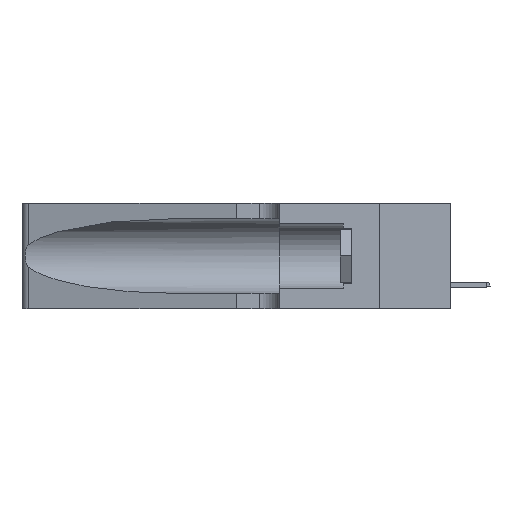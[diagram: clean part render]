
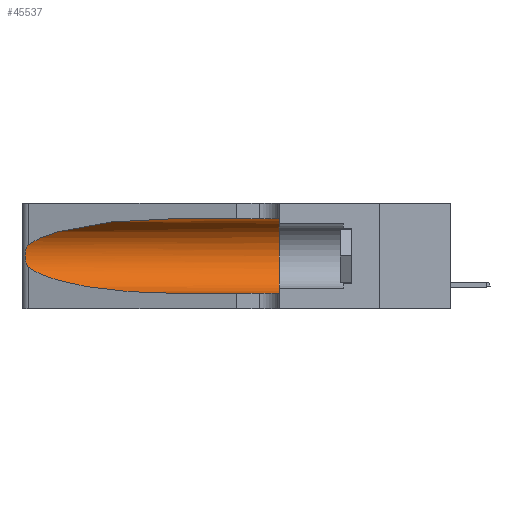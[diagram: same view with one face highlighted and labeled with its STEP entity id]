
A CAD part, left-side view. The second image highlights one B-rep face of the part: STEP entity #45537.
In plain terms, the highlighted cylindrical face has radius 3.308 mm (diameter 6.617 mm), a partial arc.
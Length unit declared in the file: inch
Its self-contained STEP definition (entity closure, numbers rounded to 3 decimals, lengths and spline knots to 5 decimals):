
#4463 = DIRECTION ( 'NONE',  ( 0., 0., -1. ) ) ;
#5229 =( BOUNDED_CURVE ( )  B_SPLINE_CURVE ( 3, ( #36028, #36274, #9947, #17600 ),
 .UNSPECIFIED., .F., .T. ) 
 B_SPLINE_CURVE_WITH_KNOTS ( ( 4, 4 ),
 ( 1.5708, 2.84003 ),
 .UNSPECIFIED. ) 
 CURVE ( )  GEOMETRIC_REPRESENTATION_ITEM ( )  RATIONAL_B_SPLINE_CURVE ( ( 1., 0.87, 0.87, 1. ) ) 
 REPRESENTATION_ITEM ( '' )  );
#5552 = CARTESIAN_POINT ( 'NONE',  ( 0.25787, 1.23484, 0.2124 ) ) ;
#5825 = VECTOR ( 'NONE', #43026, 39.37008 ) ;
#7541 = FACE_OUTER_BOUND ( 'NONE', #13295, .T. ) ;
#8801 = CIRCLE ( 'NONE', #49599, 0.13025 ) ;
#8892 = CARTESIAN_POINT ( 'NONE',  ( 0.25854, 1.2359, 0.20912 ) ) ;
#8980 = CARTESIAN_POINT ( 'NONE',  ( 0.1305, 1.61858, 0.31525 ) ) ;
#9276 = ORIENTED_EDGE ( 'NONE', *, *, #42251, .T. ) ;
#9947 = CARTESIAN_POINT ( 'NONE',  ( 0.2373, 1.15595, 0.28018 ) ) ;
#11699 = EDGE_CURVE ( 'NONE', #29842, #15133, #5229, .T. ) ;
#11769 = DIRECTION ( 'NONE',  ( 0., 0., 1. ) ) ;
#13211 = CARTESIAN_POINT ( 'NONE',  ( 0.26075, 1.23896, 0.178 ) ) ;
#13295 = EDGE_LOOP ( 'NONE', ( #16376, #9276, #49096, #31892, #16772, #41228 ) ) ;
#14584 = CARTESIAN_POINT ( 'NONE',  ( 0.1305, 0.35, 0.185 ) ) ;
#15133 = VERTEX_POINT ( 'NONE', #43805 ) ;
#16376 = ORIENTED_EDGE ( 'NONE', *, *, #11699, .T. ) ;
#16539 = CARTESIAN_POINT ( 'NONE',  ( 0.25555, 1.22994, 0.2215 ) ) ;
#16772 = ORIENTED_EDGE ( 'NONE', *, *, #38256, .F. ) ;
#17291 = CARTESIAN_POINT ( 'NONE',  ( 0.25639, 1.23184, 0.21858 ) ) ;
#17600 = CARTESIAN_POINT ( 'NONE',  ( 0.25487, 1.22718, 0.22369 ) ) ;
#18649 = LINE ( 'NONE', #45488, #50014 ) ;
#22267 = AXIS2_PLACEMENT_3D ( 'NONE', #35623, #43293, #4463 ) ;
#22501 = VERTEX_POINT ( 'NONE', #27017 ) ;
#22508 = DIRECTION ( 'NONE',  ( 0., -1., 0. ) ) ;
#24865 = VERTEX_POINT ( 'NONE', #28409 ) ;
#24983 = CARTESIAN_POINT ( 'NONE',  ( 0.26018, 1.23835, 0.19895 ) ) ;
#25232 = CARTESIAN_POINT ( 'NONE',  ( 0.26075, 1.23896, 0.19203 ) ) ;
#26278 = CARTESIAN_POINT ( 'NONE',  ( 0.18966, 0.96281, 0.05475 ) ) ;
#27017 = CARTESIAN_POINT ( 'NONE',  ( 0.1305, 0.35, 0.31525 ) ) ;
#27937 = CARTESIAN_POINT ( 'NONE',  ( 0.1305, 0.72297, 0.31525 ) ) ;
#28409 = CARTESIAN_POINT ( 'NONE',  ( 0.1305, 0.72297, 0.05475 ) ) ;
#29390 =( BOUNDED_CURVE ( )  B_SPLINE_CURVE ( 3, ( #45178, #40839, #26278, #44922 ),
 .UNSPECIFIED., .F., .T. ) 
 B_SPLINE_CURVE_WITH_KNOTS ( ( 4, 4 ),
 ( 3.44316, 4.71239 ),
 .UNSPECIFIED. ) 
 CURVE ( )  GEOMETRIC_REPRESENTATION_ITEM ( )  RATIONAL_B_SPLINE_CURVE ( ( 1., 0.87, 0.87, 1. ) ) 
 REPRESENTATION_ITEM ( '' )  );
#29842 = VERTEX_POINT ( 'NONE', #27937 ) ;
#31034 = CYLINDRICAL_SURFACE ( 'NONE', #22267, 0.13025 ) ;
#31892 = ORIENTED_EDGE ( 'NONE', *, *, #44522, .T. ) ;
#32640 = CARTESIAN_POINT ( 'NONE',  ( 0.25789, 1.23486, 0.15765 ) ) ;
#33156 = CARTESIAN_POINT ( 'NONE',  ( 0.25856, 1.23593, 0.16098 ) ) ;
#33378 = EDGE_CURVE ( 'NONE', #38504, #24865, #29390, .T. ) ;
#34775 = DIRECTION ( 'NONE',  ( 0., 1., 0. ) ) ;
#35623 = CARTESIAN_POINT ( 'NONE',  ( 0.1305, 1.61858, 0.185 ) ) ;
#36028 = CARTESIAN_POINT ( 'NONE',  ( 0.1305, 0.72297, 0.31525 ) ) ;
#36274 = CARTESIAN_POINT ( 'NONE',  ( 0.18966, 0.96281, 0.31525 ) ) ;
#36309 = LINE ( 'NONE', #8980, #5825 ) ;
#36470 = CARTESIAN_POINT ( 'NONE',  ( 0.25487, 1.22718, 0.22369 ) ) ;
#37872 = VERTEX_POINT ( 'NONE', #41565 ) ;
#38256 = EDGE_CURVE ( 'NONE', #22501, #37872, #8801, .T. ) ;
#38504 = VERTEX_POINT ( 'NONE', #41380 ) ;
#38650 = B_SPLINE_CURVE_WITH_KNOTS ( 'NONE', 3,
 ( #36470, #16539, #17291, #5552, #8892, #24983, #25232, #13211, #47744, #33156, #32640, #43878, #48753, #47993 ),
 .UNSPECIFIED., .F., .F.,
 ( 4, 2, 2, 2, 2, 2, 4 ),
 ( 0., 0.00027, 0.00053, 0.00107, 0.0016, 0.00187, 0.00214 ),
 .UNSPECIFIED. ) ;
#40839 = CARTESIAN_POINT ( 'NONE',  ( 0.2373, 1.15595, 0.08982 ) ) ;
#41228 = ORIENTED_EDGE ( 'NONE', *, *, #44194, .F. ) ;
#41380 = CARTESIAN_POINT ( 'NONE',  ( 0.25487, 1.22718, 0.14631 ) ) ;
#41565 = CARTESIAN_POINT ( 'NONE',  ( 0.1305, 0.35, 0.05475 ) ) ;
#42251 = EDGE_CURVE ( 'NONE', #15133, #38504, #38650, .T. ) ;
#43026 = DIRECTION ( 'NONE',  ( 0., -1., 0. ) ) ;
#43293 = DIRECTION ( 'NONE',  ( 0., -1., 0. ) ) ;
#43805 = CARTESIAN_POINT ( 'NONE',  ( 0.25487, 1.22718, 0.22369 ) ) ;
#43878 = CARTESIAN_POINT ( 'NONE',  ( 0.25639, 1.23186, 0.15144 ) ) ;
#44194 = EDGE_CURVE ( 'NONE', #29842, #22501, #36309, .T. ) ;
#44522 = EDGE_CURVE ( 'NONE', #24865, #37872, #18649, .T. ) ;
#44922 = CARTESIAN_POINT ( 'NONE',  ( 0.1305, 0.72297, 0.05475 ) ) ;
#45178 = CARTESIAN_POINT ( 'NONE',  ( 0.25487, 1.22718, 0.14631 ) ) ;
#45488 = CARTESIAN_POINT ( 'NONE',  ( 0.1305, 1.61858, 0.05475 ) ) ;
#45537 = ADVANCED_FACE ( 'NONE', ( #7541 ), #31034, .F. ) ;
#47744 = CARTESIAN_POINT ( 'NONE',  ( 0.26017, 1.23833, 0.17102 ) ) ;
#47993 = CARTESIAN_POINT ( 'NONE',  ( 0.25487, 1.22718, 0.14631 ) ) ;
#48753 = CARTESIAN_POINT ( 'NONE',  ( 0.25555, 1.22993, 0.14849 ) ) ;
#49096 = ORIENTED_EDGE ( 'NONE', *, *, #33378, .T. ) ;
#49599 = AXIS2_PLACEMENT_3D ( 'NONE', #14584, #34775, #11769 ) ;
#50014 = VECTOR ( 'NONE', #22508, 39.37008 ) ;
